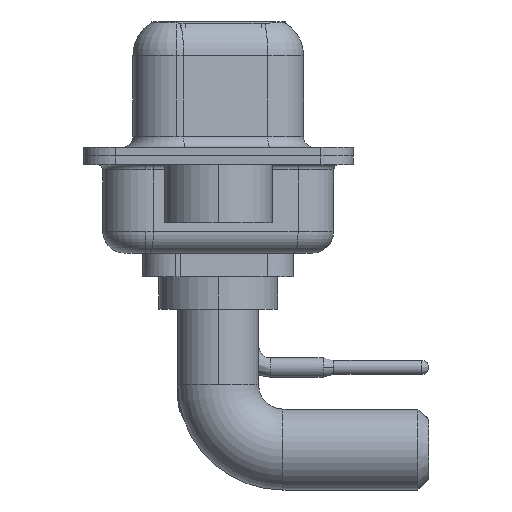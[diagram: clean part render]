
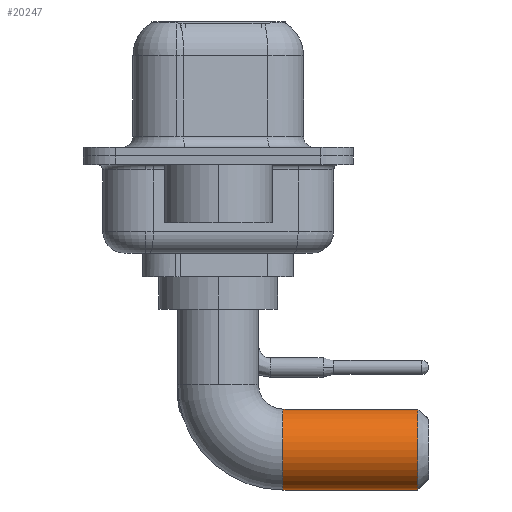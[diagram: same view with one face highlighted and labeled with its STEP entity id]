
A CAD part, left-side view. The second image highlights one B-rep face of the part: STEP entity #20247.
In plain terms, the highlighted cylindrical face has radius 1.875 mm (diameter 3.75 mm), a partial arc.
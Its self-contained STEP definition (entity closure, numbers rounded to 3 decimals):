
#40 = FACE_OUTER_BOUND ( 'NONE', #5863, .T. ) ;
#2710 = DIRECTION ( 'NONE',  ( 0., -1., 0. ) ) ;
#3846 = ORIENTED_EDGE ( 'NONE', *, *, #15534, .T. ) ;
#3996 = VECTOR ( 'NONE', #4404, 1000. ) ;
#4154 = DIRECTION ( 'NONE',  ( 0., 0., -1. ) ) ;
#4404 = DIRECTION ( 'NONE',  ( 0., -1., 0. ) ) ;
#5158 = DIRECTION ( 'NONE',  ( 0., -1., 0. ) ) ;
#5335 = CARTESIAN_POINT ( 'NONE',  ( 0., -3., -4.625 ) ) ;
#5863 = EDGE_LOOP ( 'NONE', ( #14452, #8013, #3846, #13263 ) ) ;
#6013 = AXIS2_PLACEMENT_3D ( 'NONE', #23235, #9323, #4154 ) ;
#7533 = LINE ( 'NONE', #22837, #12444 ) ;
#8013 = ORIENTED_EDGE ( 'NONE', *, *, #20884, .T. ) ;
#8178 = CARTESIAN_POINT ( 'NONE',  ( 0., -3., -4.625 ) ) ;
#8550 = DIRECTION ( 'NONE',  ( 0., 1., 0. ) ) ;
#8855 = CARTESIAN_POINT ( 'NONE',  ( 0., -9.25, -4.625 ) ) ;
#9323 = DIRECTION ( 'NONE',  ( 0., -1., 0. ) ) ;
#10753 = EDGE_CURVE ( 'NONE', #17115, #13656, #23484, .T. ) ;
#11484 = CARTESIAN_POINT ( 'NONE',  ( 0., -3., -8.375 ) ) ;
#11844 = CYLINDRICAL_SURFACE ( 'NONE', #6013, 1.875 ) ;
#12444 = VECTOR ( 'NONE', #5158, 1000. ) ;
#12467 = DIRECTION ( 'NONE',  ( 0., 0., -1. ) ) ;
#13263 = ORIENTED_EDGE ( 'NONE', *, *, #10753, .T. ) ;
#13656 = VERTEX_POINT ( 'NONE', #8855 ) ;
#13804 = VERTEX_POINT ( 'NONE', #11484 ) ;
#13875 = LINE ( 'NONE', #8178, #3996 ) ;
#14303 = DIRECTION ( 'NONE',  ( -1., 0., 0. ) ) ;
#14452 = ORIENTED_EDGE ( 'NONE', *, *, #15249, .F. ) ;
#15249 = EDGE_CURVE ( 'NONE', #21136, #13656, #13875, .T. ) ;
#15534 = EDGE_CURVE ( 'NONE', #13804, #17115, #7533, .T. ) ;
#15917 = AXIS2_PLACEMENT_3D ( 'NONE', #17974, #8550, #12467 ) ;
#16508 = CIRCLE ( 'NONE', #23674, 1.875 ) ;
#17115 = VERTEX_POINT ( 'NONE', #17263 ) ;
#17263 = CARTESIAN_POINT ( 'NONE',  ( 0., -9.25, -8.375 ) ) ;
#17974 = CARTESIAN_POINT ( 'NONE',  ( 0., -9.25, -6.5 ) ) ;
#20247 = ADVANCED_FACE ( 'NONE', ( #40 ), #11844, .T. ) ;
#20884 = EDGE_CURVE ( 'NONE', #21136, #13804, #16508, .T. ) ;
#21136 = VERTEX_POINT ( 'NONE', #5335 ) ;
#21774 = CARTESIAN_POINT ( 'NONE',  ( 0., -3., -6.5 ) ) ;
#22837 = CARTESIAN_POINT ( 'NONE',  ( 0., -3., -8.375 ) ) ;
#23235 = CARTESIAN_POINT ( 'NONE',  ( 0., -3., -6.5 ) ) ;
#23484 = CIRCLE ( 'NONE', #15917, 1.875 ) ;
#23674 = AXIS2_PLACEMENT_3D ( 'NONE', #21774, #2710, #14303 ) ;
